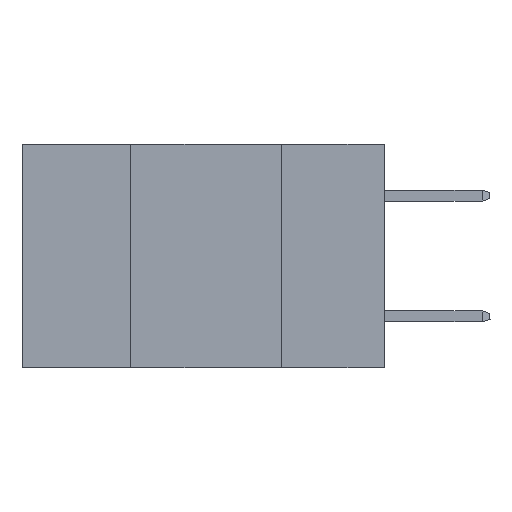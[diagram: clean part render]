
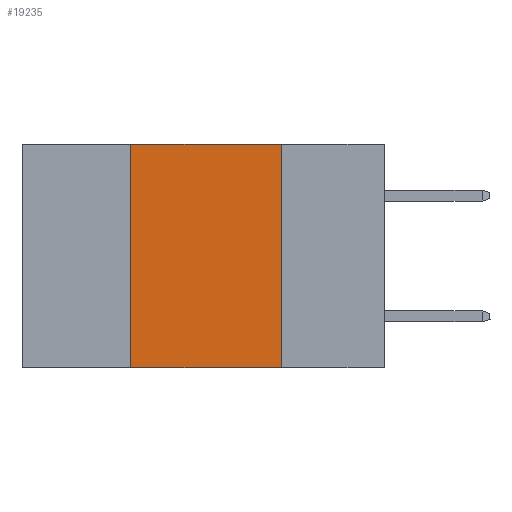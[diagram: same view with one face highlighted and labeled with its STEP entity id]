
A CAD part, left-side view. The second image highlights one B-rep face of the part: STEP entity #19235.
In plain terms, the highlighted planar face has unit normal (-1, 0, 0).
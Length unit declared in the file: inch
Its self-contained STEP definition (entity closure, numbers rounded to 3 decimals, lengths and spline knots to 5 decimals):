
#1069 = DIRECTION ( 'NONE',  ( 0., 0., 1. ) ) ;
#1550 = ORIENTED_EDGE ( 'NONE', *, *, #9390, .F. ) ;
#1711 = VECTOR ( 'NONE', #1069, 39.37008 ) ;
#2647 = FACE_OUTER_BOUND ( 'NONE', #21022, .T. ) ;
#2744 = CARTESIAN_POINT ( 'NONE',  ( 0., 0.6, 0. ) ) ;
#3166 = ORIENTED_EDGE ( 'NONE', *, *, #3842, .F. ) ;
#3542 = LINE ( 'NONE', #11991, #13657 ) ;
#3695 = CARTESIAN_POINT ( 'NONE',  ( 0., 0.6, -0.37 ) ) ;
#3842 = EDGE_CURVE ( 'NONE', #17101, #23296, #14244, .T. ) ;
#4407 = VERTEX_POINT ( 'NONE', #13350 ) ;
#5480 = ORIENTED_EDGE ( 'NONE', *, *, #13523, .F. ) ;
#5687 = DIRECTION ( 'NONE',  ( 0., -1., 0. ) ) ;
#5737 = CARTESIAN_POINT ( 'NONE',  ( 0., 0.17, 0. ) ) ;
#7646 = DIRECTION ( 'NONE',  ( 0., 0., -1. ) ) ;
#7652 = LINE ( 'NONE', #13119, #1711 ) ;
#9390 = EDGE_CURVE ( 'NONE', #25609, #17101, #7652, .T. ) ;
#11991 = CARTESIAN_POINT ( 'NONE',  ( 0., 0.17, -0.37 ) ) ;
#12966 = LINE ( 'NONE', #3695, #17008 ) ;
#13119 = CARTESIAN_POINT ( 'NONE',  ( 0., 0.42, -0.37 ) ) ;
#13350 = CARTESIAN_POINT ( 'NONE',  ( 0., 0.17, -0.37 ) ) ;
#13523 = EDGE_CURVE ( 'NONE', #23296, #4407, #3542, .T. ) ;
#13657 = VECTOR ( 'NONE', #14039, 39.37008 ) ;
#13862 = DIRECTION ( 'NONE',  ( 0., -1., 0. ) ) ;
#14039 = DIRECTION ( 'NONE',  ( 0., 0., -1. ) ) ;
#14219 = AXIS2_PLACEMENT_3D ( 'NONE', #25540, #19667, #7646 ) ;
#14244 = LINE ( 'NONE', #2744, #24147 ) ;
#15780 = CARTESIAN_POINT ( 'NONE',  ( 0., 0.42, -0.37 ) ) ;
#16323 = ORIENTED_EDGE ( 'NONE', *, *, #22482, .T. ) ;
#17008 = VECTOR ( 'NONE', #13862, 39.37008 ) ;
#17101 = VERTEX_POINT ( 'NONE', #25459 ) ;
#17679 = PLANE ( 'NONE',  #14219 ) ;
#19235 = ADVANCED_FACE ( 'NONE', ( #2647 ), #17679, .F. ) ;
#19667 = DIRECTION ( 'NONE',  ( 1., 0., 0. ) ) ;
#21022 = EDGE_LOOP ( 'NONE', ( #5480, #3166, #1550, #16323 ) ) ;
#22482 = EDGE_CURVE ( 'NONE', #25609, #4407, #12966, .T. ) ;
#23296 = VERTEX_POINT ( 'NONE', #5737 ) ;
#24147 = VECTOR ( 'NONE', #5687, 39.37008 ) ;
#25459 = CARTESIAN_POINT ( 'NONE',  ( 0., 0.42, 0. ) ) ;
#25540 = CARTESIAN_POINT ( 'NONE',  ( 0., 0.6, 0. ) ) ;
#25609 = VERTEX_POINT ( 'NONE', #15780 ) ;
